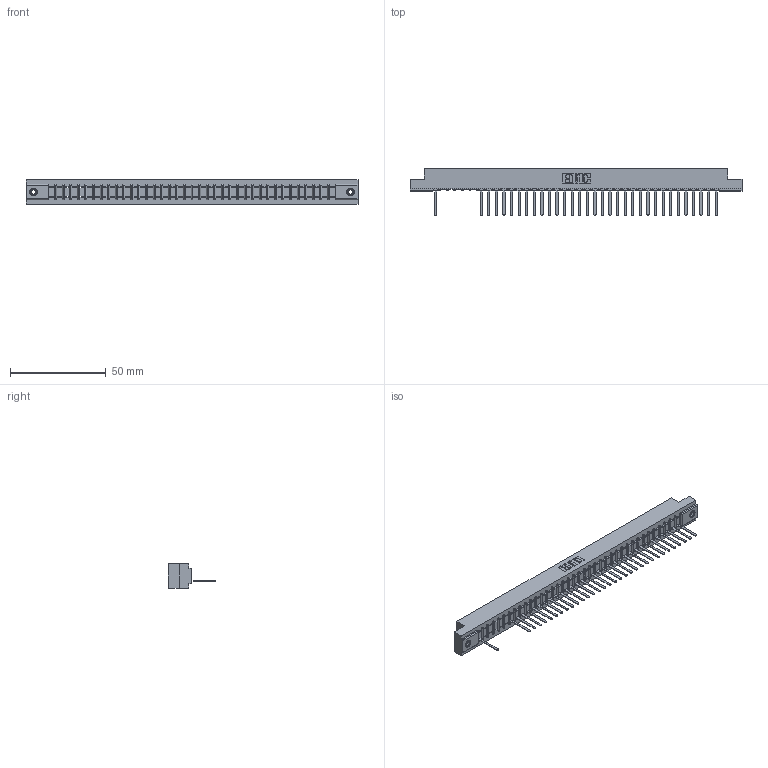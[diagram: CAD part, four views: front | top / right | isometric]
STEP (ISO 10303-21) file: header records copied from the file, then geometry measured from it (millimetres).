
FILE_DESCRIPTION (( 'STEP AP203' ), '1' );
FILE_NAME ('357-038-541-108.STEP', '2018-08-10T09:16:22', ( '' ), ( '' ), 'SwSTEP 2.0', 'SolidWorks 2016', '' );
FILE_SCHEMA (( 'CONFIG_CONTROL_DESIGN' ));
Length unit declared in the file: inch
Products named in the file (4): 307 Part_.156 Dia Mounting Holes; 307-290-002_541; 345-250-001_345-250-003-102; 357-038-541-108
Assembly tree (36 placements, depth 2):
  357-038-541-108
    307 Part_.156 Dia Mounting Holes
    307-290-002_541  x33
    345-250-001_345-250-003-102  x2
Bounding box: 173.58 x 24.59 x 12.7 mm (x, y, z)
Volume: 18487.7 mm3; surface area: 22850.3 mm2
Topology: 36 solids, 36 shells, 2759 faces, 8435 edges, 5510 vertices
Faces by surface type: plane 1647, cylinder 1018, sphere 78, cone 12, torus 4
Entity records: 34813 total; most frequent: CARTESIAN_POINT 5874, ORIENTED_EDGE 5862, DIRECTION 5713, EDGE_CURVE 2931, VECTOR 2243, LINE 2243, VERTEX_POINT 1896, AXIS2_PLACEMENT_3D 1735
